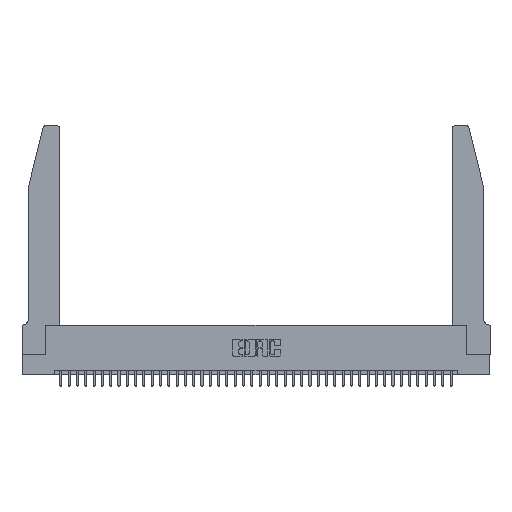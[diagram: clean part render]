
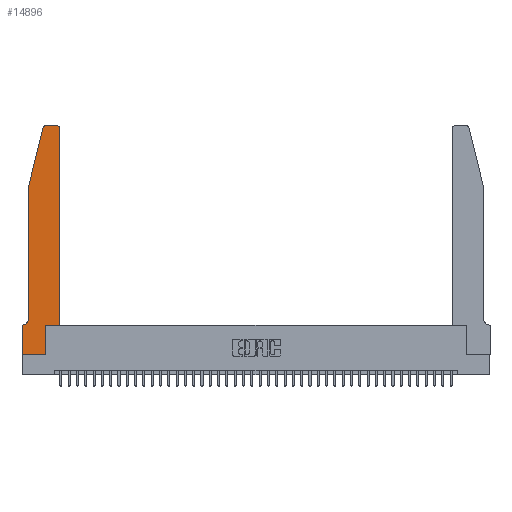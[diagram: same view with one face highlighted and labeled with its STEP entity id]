
A CAD part, top view. The second image highlights one B-rep face of the part: STEP entity #14896.
In plain terms, the highlighted planar face has unit normal (0, 0, 1).
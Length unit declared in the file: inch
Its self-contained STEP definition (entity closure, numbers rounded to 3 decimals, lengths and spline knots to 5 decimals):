
#2 = EDGE_CURVE ( 'NONE', #2867, #39922, #38001, .T. ) ;
#317 = CARTESIAN_POINT ( 'NONE',  ( 0.4505, 2.72, 0.37 ) ) ;
#695 = LINE ( 'NONE', #35278, #40416 ) ;
#1419 = AXIS2_PLACEMENT_3D ( 'NONE', #29712, #10508, #32915 ) ;
#1983 = ORIENTED_EDGE ( 'NONE', *, *, #40319, .T. ) ;
#2064 = ORIENTED_EDGE ( 'NONE', *, *, #17574, .T. ) ;
#2164 = CARTESIAN_POINT ( 'NONE',  ( 0., 0., 0.37 ) ) ;
#2664 = DIRECTION ( 'NONE',  ( 0., 0., -1. ) ) ;
#2867 = VERTEX_POINT ( 'NONE', #317 ) ;
#3210 = VERTEX_POINT ( 'NONE', #8443 ) ;
#3230 = DIRECTION ( 'NONE',  ( 0., 1., 0. ) ) ;
#3789 = CARTESIAN_POINT ( 'NONE',  ( 0.0055, 0.35, 0.37 ) ) ;
#4059 = EDGE_CURVE ( 'NONE', #7447, #40143, #26222, .T. ) ;
#4205 = VERTEX_POINT ( 'NONE', #3789 ) ;
#6091 = EDGE_CURVE ( 'NONE', #3210, #7447, #26309, .T. ) ;
#6117 = CIRCLE ( 'NONE', #40263, 0.07 ) ;
#6206 = VERTEX_POINT ( 'NONE', #37852 ) ;
#6226 = ORIENTED_EDGE ( 'NONE', *, *, #10793, .T. ) ;
#6335 = VECTOR ( 'NONE', #22209, 39.37008 ) ;
#6367 = VECTOR ( 'NONE', #15185, 39.37008 ) ;
#7285 = CARTESIAN_POINT ( 'NONE',  ( 0., 0.35, 0.37 ) ) ;
#7447 = VERTEX_POINT ( 'NONE', #34857 ) ;
#7468 = LINE ( 'NONE', #29456, #15019 ) ;
#7862 = VERTEX_POINT ( 'NONE', #41130 ) ;
#8443 = CARTESIAN_POINT ( 'NONE',  ( 0., 0., 0.37 ) ) ;
#8712 = CARTESIAN_POINT ( 'NONE',  ( 0.2865, 0.35, 0.37 ) ) ;
#8770 = EDGE_LOOP ( 'NONE', ( #1983, #10674, #24278, #2064, #38812, #6226, #16824, #35861, #8812, #21397, #9781, #23364 ) ) ;
#8812 = ORIENTED_EDGE ( 'NONE', *, *, #4059, .T. ) ;
#9427 = CARTESIAN_POINT ( 'NONE',  ( 0.2605, 2.75, 0.37 ) ) ;
#9555 = DIRECTION ( 'NONE',  ( 1., 0., 0. ) ) ;
#9781 = ORIENTED_EDGE ( 'NONE', *, *, #11950, .T. ) ;
#10508 = DIRECTION ( 'NONE',  ( 0., 0., 1. ) ) ;
#10588 = AXIS2_PLACEMENT_3D ( 'NONE', #11887, #15092, #37500 ) ;
#10674 = ORIENTED_EDGE ( 'NONE', *, *, #19675, .T. ) ;
#10793 = EDGE_CURVE ( 'NONE', #4205, #19129, #20475, .T. ) ;
#10916 = VECTOR ( 'NONE', #19853, 39.37008 ) ;
#11084 = AXIS2_PLACEMENT_3D ( 'NONE', #25799, #12777, #9555 ) ;
#11887 = CARTESIAN_POINT ( 'NONE',  ( 0., 0.35, 0.37 ) ) ;
#11950 = EDGE_CURVE ( 'NONE', #25816, #2867, #40859, .T. ) ;
#12777 = DIRECTION ( 'NONE',  ( 0., 0., 1. ) ) ;
#13334 = VECTOR ( 'NONE', #29722, 39.37008 ) ;
#14896 = ADVANCED_FACE ( 'NONE', ( #26512 ), #40551, .T. ) ;
#15019 = VECTOR ( 'NONE', #29729, 39.37008 ) ;
#15092 = DIRECTION ( 'NONE',  ( 0., 0., 1. ) ) ;
#15185 = DIRECTION ( 'NONE',  ( 0., -1., 0. ) ) ;
#16824 = ORIENTED_EDGE ( 'NONE', *, *, #28589, .T. ) ;
#17574 = EDGE_CURVE ( 'NONE', #6206, #30876, #22810, .T. ) ;
#17978 = LINE ( 'NONE', #2164, #6367 ) ;
#18709 = VECTOR ( 'NONE', #3230, 39.37008 ) ;
#18975 = CARTESIAN_POINT ( 'NONE',  ( 0.4505, 0.35, 0.37 ) ) ;
#19129 = VERTEX_POINT ( 'NONE', #7285 ) ;
#19675 = EDGE_CURVE ( 'NONE', #39359, #7862, #30001, .T. ) ;
#19853 = DIRECTION ( 'NONE',  ( -1., 0., 0. ) ) ;
#20475 = LINE ( 'NONE', #35785, #10916 ) ;
#21397 = ORIENTED_EDGE ( 'NONE', *, *, #27654, .T. ) ;
#22033 = CARTESIAN_POINT ( 'NONE',  ( 0.0055, 0.42, 0.37 ) ) ;
#22209 = DIRECTION ( 'NONE',  ( -1., 0., 0. ) ) ;
#22389 = VECTOR ( 'NONE', #25788, 39.37008 ) ;
#22810 = LINE ( 'NONE', #35310, #22389 ) ;
#23364 = ORIENTED_EDGE ( 'NONE', *, *, #2, .T. ) ;
#23478 = LINE ( 'NONE', #9427, #6335 ) ;
#24278 = ORIENTED_EDGE ( 'NONE', *, *, #29027, .T. ) ;
#25218 = DIRECTION ( 'NONE',  ( -1., 0., 0. ) ) ;
#25788 = DIRECTION ( 'NONE',  ( 0., -1., 0. ) ) ;
#25799 = CARTESIAN_POINT ( 'NONE',  ( 0.4205, 2.72, 0.37 ) ) ;
#25816 = VERTEX_POINT ( 'NONE', #18975 ) ;
#26222 = LINE ( 'NONE', #38488, #18709 ) ;
#26309 = LINE ( 'NONE', #40353, #41300 ) ;
#26512 = FACE_OUTER_BOUND ( 'NONE', #8770, .T. ) ;
#26626 = CARTESIAN_POINT ( 'NONE',  ( 0.4505, 0.35, 0.37 ) ) ;
#26952 = CARTESIAN_POINT ( 'NONE',  ( 0.4205, 2.75, 0.37 ) ) ;
#27654 = EDGE_CURVE ( 'NONE', #40143, #25816, #7468, .T. ) ;
#28589 = EDGE_CURVE ( 'NONE', #19129, #3210, #17978, .T. ) ;
#29027 = EDGE_CURVE ( 'NONE', #7862, #6206, #695, .T. ) ;
#29456 = CARTESIAN_POINT ( 'NONE',  ( 0.4505, 0.35, 0.37 ) ) ;
#29712 = CARTESIAN_POINT ( 'NONE',  ( 0.284, 2.72, 0.37 ) ) ;
#29722 = DIRECTION ( 'NONE',  ( 0., 1., 0. ) ) ;
#29729 = DIRECTION ( 'NONE',  ( 1., 0., 0. ) ) ;
#30001 = CIRCLE ( 'NONE', #1419, 0.03 ) ;
#30876 = VERTEX_POINT ( 'NONE', #38606 ) ;
#32915 = DIRECTION ( 'NONE',  ( 1., 0., 0. ) ) ;
#33273 = CARTESIAN_POINT ( 'NONE',  ( 0.284, 2.75, 0.37 ) ) ;
#34105 = DIRECTION ( 'NONE',  ( 1., 0., 0. ) ) ;
#34857 = CARTESIAN_POINT ( 'NONE',  ( 0.2865, 0., 0.37 ) ) ;
#35278 = CARTESIAN_POINT ( 'NONE',  ( 0.0755, 2., 0.37 ) ) ;
#35310 = CARTESIAN_POINT ( 'NONE',  ( 0.0755, 2., 0.37 ) ) ;
#35785 = CARTESIAN_POINT ( 'NONE',  ( 0.0755, 0.35, 0.37 ) ) ;
#35861 = ORIENTED_EDGE ( 'NONE', *, *, #6091, .T. ) ;
#37007 = EDGE_CURVE ( 'NONE', #30876, #4205, #6117, .T. ) ;
#37500 = DIRECTION ( 'NONE',  ( 1., 0., 0. ) ) ;
#37852 = CARTESIAN_POINT ( 'NONE',  ( 0.0755, 2., 0.37 ) ) ;
#38001 = CIRCLE ( 'NONE', #11084, 0.03 ) ;
#38469 = DIRECTION ( 'NONE',  ( -0.239, -0.971, 0. ) ) ;
#38488 = CARTESIAN_POINT ( 'NONE',  ( 0.2865, 0.35, 0.37 ) ) ;
#38606 = CARTESIAN_POINT ( 'NONE',  ( 0.0755, 0.42, 0.37 ) ) ;
#38812 = ORIENTED_EDGE ( 'NONE', *, *, #37007, .T. ) ;
#39359 = VERTEX_POINT ( 'NONE', #33273 ) ;
#39922 = VERTEX_POINT ( 'NONE', #26952 ) ;
#40143 = VERTEX_POINT ( 'NONE', #8712 ) ;
#40263 = AXIS2_PLACEMENT_3D ( 'NONE', #22033, #2664, #25218 ) ;
#40319 = EDGE_CURVE ( 'NONE', #39922, #39359, #23478, .T. ) ;
#40353 = CARTESIAN_POINT ( 'NONE',  ( 0., 0., 0.37 ) ) ;
#40416 = VECTOR ( 'NONE', #38469, 39.37008 ) ;
#40551 = PLANE ( 'NONE',  #10588 ) ;
#40859 = LINE ( 'NONE', #26626, #13334 ) ;
#41130 = CARTESIAN_POINT ( 'NONE',  ( 0.25487, 2.72718, 0.37 ) ) ;
#41300 = VECTOR ( 'NONE', #34105, 39.37008 ) ;
